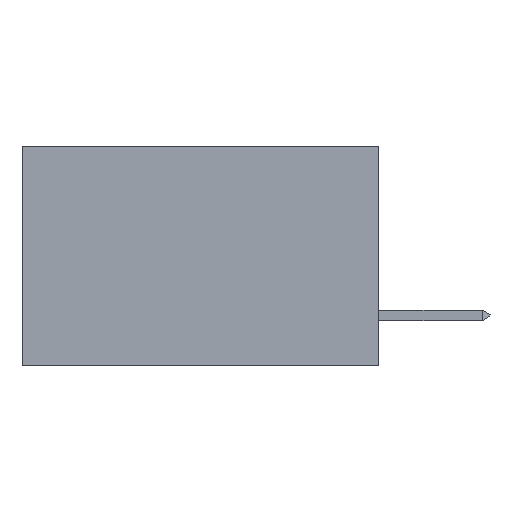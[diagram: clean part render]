
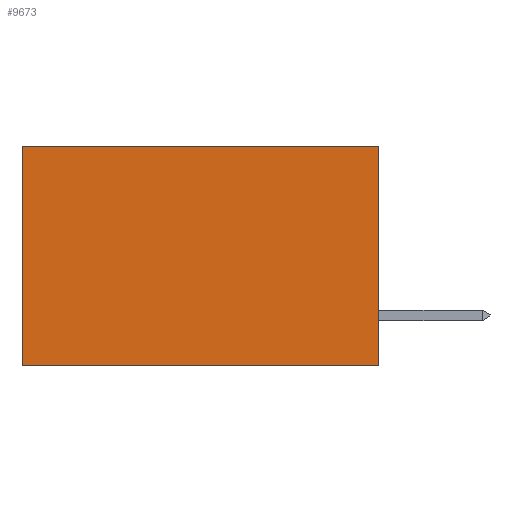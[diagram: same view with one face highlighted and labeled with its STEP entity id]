
A CAD part, left-side view. The second image highlights one B-rep face of the part: STEP entity #9673.
In plain terms, the highlighted planar face has unit normal (-1, 0, 0).
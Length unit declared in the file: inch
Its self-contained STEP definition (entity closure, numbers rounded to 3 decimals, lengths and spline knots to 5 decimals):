
#145 = VECTOR ( 'NONE', #2940, 39.37008 ) ;
#349 = FACE_OUTER_BOUND ( 'NONE', #13718, .T. ) ;
#700 = ORIENTED_EDGE ( 'NONE', *, *, #14667, .T. ) ;
#939 = DIRECTION ( 'NONE',  ( 0., 1., 0. ) ) ;
#1056 = VERTEX_POINT ( 'NONE', #2980 ) ;
#1088 = CARTESIAN_POINT ( 'NONE',  ( 0.298, 0.6, 0. ) ) ;
#1546 = DIRECTION ( 'NONE',  ( 0., 0., -1. ) ) ;
#1881 = EDGE_CURVE ( 'NONE', #1056, #9216, #11320, .T. ) ;
#2827 = VECTOR ( 'NONE', #1546, 39.37008 ) ;
#2940 = DIRECTION ( 'NONE',  ( 0., 0., -1. ) ) ;
#2980 = CARTESIAN_POINT ( 'NONE',  ( 0.298, 0., -0.37 ) ) ;
#3064 = DIRECTION ( 'NONE',  ( 0., 0., -1. ) ) ;
#3147 = PLANE ( 'NONE',  #11500 ) ;
#3734 = ORIENTED_EDGE ( 'NONE', *, *, #1881, .F. ) ;
#4098 = LINE ( 'NONE', #11567, #16486 ) ;
#4829 = EDGE_CURVE ( 'NONE', #20079, #1056, #14062, .T. ) ;
#6893 = CARTESIAN_POINT ( 'NONE',  ( 0.298, 0., 0. ) ) ;
#6980 = VERTEX_POINT ( 'NONE', #15456 ) ;
#7448 = ORIENTED_EDGE ( 'NONE', *, *, #4829, .F. ) ;
#7777 = EDGE_CURVE ( 'NONE', #6980, #9216, #12832, .T. ) ;
#9216 = VERTEX_POINT ( 'NONE', #18613 ) ;
#9673 = ADVANCED_FACE ( 'NONE', ( #349 ), #3147, .F. ) ;
#11320 = LINE ( 'NONE', #12481, #11917 ) ;
#11500 = AXIS2_PLACEMENT_3D ( 'NONE', #6893, #18055, #3064 ) ;
#11567 = CARTESIAN_POINT ( 'NONE',  ( 0.298, 0., 0. ) ) ;
#11917 = VECTOR ( 'NONE', #939, 39.37008 ) ;
#12481 = CARTESIAN_POINT ( 'NONE',  ( 0.298, 0., -0.37 ) ) ;
#12832 = LINE ( 'NONE', #1088, #145 ) ;
#13718 = EDGE_LOOP ( 'NONE', ( #22277, #3734, #7448, #700 ) ) ;
#14062 = LINE ( 'NONE', #20598, #2827 ) ;
#14667 = EDGE_CURVE ( 'NONE', #20079, #6980, #4098, .T. ) ;
#15456 = CARTESIAN_POINT ( 'NONE',  ( 0.298, 0.6, 0. ) ) ;
#16486 = VECTOR ( 'NONE', #18992, 39.37008 ) ;
#18055 = DIRECTION ( 'NONE',  ( 1., 0., 0. ) ) ;
#18613 = CARTESIAN_POINT ( 'NONE',  ( 0.298, 0.6, -0.37 ) ) ;
#18992 = DIRECTION ( 'NONE',  ( 0., 1., 0. ) ) ;
#19714 = CARTESIAN_POINT ( 'NONE',  ( 0.298, 0., 0. ) ) ;
#20079 = VERTEX_POINT ( 'NONE', #19714 ) ;
#20598 = CARTESIAN_POINT ( 'NONE',  ( 0.298, 0., 0. ) ) ;
#22277 = ORIENTED_EDGE ( 'NONE', *, *, #7777, .T. ) ;
